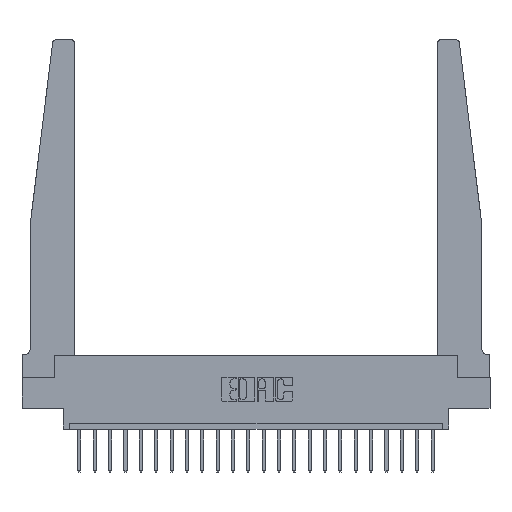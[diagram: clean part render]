
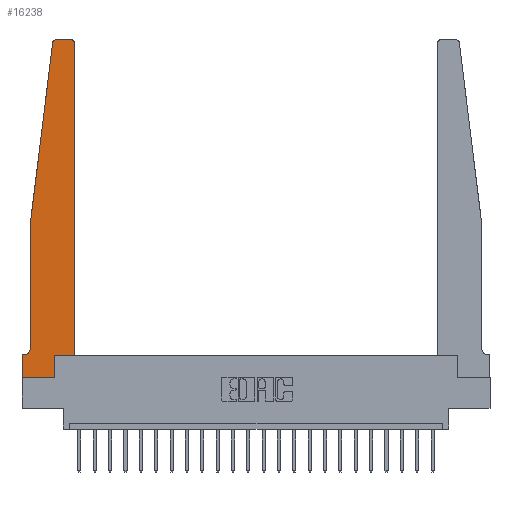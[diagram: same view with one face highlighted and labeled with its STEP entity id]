
A CAD part, top view. The second image highlights one B-rep face of the part: STEP entity #16238.
In plain terms, the highlighted planar face has unit normal (0, 0, 1).
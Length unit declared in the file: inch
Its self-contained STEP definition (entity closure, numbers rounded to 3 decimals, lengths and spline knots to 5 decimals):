
#198 = CARTESIAN_POINT ( 'NONE',  ( 0.015, 0.2375, 0.37 ) ) ;
#364 = CARTESIAN_POINT ( 'NONE',  ( 0.015, 0.1875, 0.37 ) ) ;
#538 = CARTESIAN_POINT ( 'NONE',  ( 0., 0., 0.37 ) ) ;
#600 = VECTOR ( 'NONE', #3286, 39.37008 ) ;
#659 = DIRECTION ( 'NONE',  ( -1., 0., 0. ) ) ;
#666 = CARTESIAN_POINT ( 'NONE',  ( 0.2605, 0.18, 0.37 ) ) ;
#715 = DIRECTION ( 'NONE',  ( 0., 0., 1. ) ) ;
#872 = ORIENTED_EDGE ( 'NONE', *, *, #12232, .T. ) ;
#929 = ORIENTED_EDGE ( 'NONE', *, *, #10654, .T. ) ;
#946 = CARTESIAN_POINT ( 'NONE',  ( 0.425, 0.18, 0.37 ) ) ;
#1233 = CARTESIAN_POINT ( 'NONE',  ( 0., 0., 0.37 ) ) ;
#1246 = CIRCLE ( 'NONE', #12226, 0.03 ) ;
#1289 = VECTOR ( 'NONE', #13585, 39.37008 ) ;
#1361 = CARTESIAN_POINT ( 'NONE',  ( 0.395, 2.75, 0.37 ) ) ;
#2109 = CARTESIAN_POINT ( 'NONE',  ( 0.065, 1.25, 0.37 ) ) ;
#2421 = DIRECTION ( 'NONE',  ( 1., 0., 0. ) ) ;
#2498 = DIRECTION ( 'NONE',  ( 0., 1., 0. ) ) ;
#2723 = ORIENTED_EDGE ( 'NONE', *, *, #3501, .T. ) ;
#3271 = CARTESIAN_POINT ( 'NONE',  ( 0.065, 1.25, 0.37 ) ) ;
#3286 = DIRECTION ( 'NONE',  ( 1., 0., 0. ) ) ;
#3501 = EDGE_CURVE ( 'NONE', #21080, #10775, #15341, .T. ) ;
#3715 = CARTESIAN_POINT ( 'NONE',  ( 0.395, 2.72, 0.37 ) ) ;
#3867 = DIRECTION ( 'NONE',  ( 0., 0., -1. ) ) ;
#3941 = EDGE_CURVE ( 'NONE', #10124, #15934, #20706, .T. ) ;
#4116 = CARTESIAN_POINT ( 'NONE',  ( 0.2605, 0., 0.37 ) ) ;
#4182 = CIRCLE ( 'NONE', #19936, 0.03 ) ;
#4541 = VECTOR ( 'NONE', #10244, 39.37008 ) ;
#4709 = ORIENTED_EDGE ( 'NONE', *, *, #15875, .T. ) ;
#4868 = CARTESIAN_POINT ( 'NONE',  ( 0.425, 0.18, 0.37 ) ) ;
#4977 = CARTESIAN_POINT ( 'NONE',  ( 0.425, 0.18, 0.37 ) ) ;
#5013 = DIRECTION ( 'NONE',  ( 0., -1., 0. ) ) ;
#5187 = DIRECTION ( 'NONE',  ( 1., 0., 0. ) ) ;
#5736 = CARTESIAN_POINT ( 'NONE',  ( 0.065, 0.2375, 0.37 ) ) ;
#5769 = EDGE_CURVE ( 'NONE', #15934, #6411, #4182, .T. ) ;
#5777 = CARTESIAN_POINT ( 'NONE',  ( 0.25, 2.75, 0.37 ) ) ;
#6395 = EDGE_CURVE ( 'NONE', #18772, #19838, #18056, .T. ) ;
#6411 = VERTEX_POINT ( 'NONE', #1361 ) ;
#6445 = EDGE_CURVE ( 'NONE', #16735, #21080, #10162, .T. ) ;
#6631 = ORIENTED_EDGE ( 'NONE', *, *, #19994, .T. ) ;
#6645 = VERTEX_POINT ( 'NONE', #15446 ) ;
#6826 = ORIENTED_EDGE ( 'NONE', *, *, #6395, .T. ) ;
#6922 = VECTOR ( 'NONE', #19562, 39.37008 ) ;
#7030 = EDGE_LOOP ( 'NONE', ( #4709, #20001, #929, #6631, #14098, #20085, #2723, #872, #6826, #9882, #8824, #18214 ) ) ;
#7211 = EDGE_CURVE ( 'NONE', #6645, #12249, #1246, .T. ) ;
#7307 = CARTESIAN_POINT ( 'NONE',  ( 0.065, 1.25, 0.37 ) ) ;
#8092 = CARTESIAN_POINT ( 'NONE',  ( 0., 0.1875, 0.37 ) ) ;
#8280 = EDGE_CURVE ( 'NONE', #19838, #10124, #18859, .T. ) ;
#8742 = DIRECTION ( 'NONE',  ( 0., 0., 1. ) ) ;
#8824 = ORIENTED_EDGE ( 'NONE', *, *, #3941, .T. ) ;
#9199 = EDGE_CURVE ( 'NONE', #10140, #16735, #17392, .T. ) ;
#9515 = AXIS2_PLACEMENT_3D ( 'NONE', #15859, #17453, #12198 ) ;
#9882 = ORIENTED_EDGE ( 'NONE', *, *, #8280, .T. ) ;
#9990 = VERTEX_POINT ( 'NONE', #2109 ) ;
#10124 = VERTEX_POINT ( 'NONE', #946 ) ;
#10140 = VERTEX_POINT ( 'NONE', #5736 ) ;
#10162 = LINE ( 'NONE', #18993, #10709 ) ;
#10244 = DIRECTION ( 'NONE',  ( 0., -1., 0. ) ) ;
#10272 = DIRECTION ( 'NONE',  ( -1., 0., 0. ) ) ;
#10654 = EDGE_CURVE ( 'NONE', #12249, #9990, #12238, .T. ) ;
#10709 = VECTOR ( 'NONE', #10272, 39.37008 ) ;
#10775 = VERTEX_POINT ( 'NONE', #538 ) ;
#10818 = FACE_OUTER_BOUND ( 'NONE', #7030, .T. ) ;
#11543 = AXIS2_PLACEMENT_3D ( 'NONE', #198, #3867, #659 ) ;
#11812 = VECTOR ( 'NONE', #2498, 39.37008 ) ;
#11984 = DIRECTION ( 'NONE',  ( 0., 1., 0. ) ) ;
#12198 = DIRECTION ( 'NONE',  ( 1., 0., 0. ) ) ;
#12226 = AXIS2_PLACEMENT_3D ( 'NONE', #19854, #715, #2421 ) ;
#12232 = EDGE_CURVE ( 'NONE', #10775, #18772, #18986, .T. ) ;
#12238 = LINE ( 'NONE', #7307, #13034 ) ;
#12249 = VERTEX_POINT ( 'NONE', #22535 ) ;
#12424 = PLANE ( 'NONE',  #9515 ) ;
#13034 = VECTOR ( 'NONE', #17498, 39.37008 ) ;
#13585 = DIRECTION ( 'NONE',  ( 1., 0., 0. ) ) ;
#14098 = ORIENTED_EDGE ( 'NONE', *, *, #9199, .T. ) ;
#14279 = LINE ( 'NONE', #5777, #6922 ) ;
#14568 = VECTOR ( 'NONE', #11984, 39.37008 ) ;
#15341 = LINE ( 'NONE', #17277, #18631 ) ;
#15446 = CARTESIAN_POINT ( 'NONE',  ( 0.27653, 2.75, 0.37 ) ) ;
#15513 = LINE ( 'NONE', #3271, #4541 ) ;
#15859 = CARTESIAN_POINT ( 'NONE',  ( 0., 0.1875, 0.37 ) ) ;
#15875 = EDGE_CURVE ( 'NONE', #6411, #6645, #14279, .T. ) ;
#15934 = VERTEX_POINT ( 'NONE', #16447 ) ;
#16238 = ADVANCED_FACE ( 'NONE', ( #10818 ), #12424, .T. ) ;
#16443 = CARTESIAN_POINT ( 'NONE',  ( 0.2605, 0.18, 0.37 ) ) ;
#16447 = CARTESIAN_POINT ( 'NONE',  ( 0.425, 2.72, 0.37 ) ) ;
#16735 = VERTEX_POINT ( 'NONE', #364 ) ;
#17277 = CARTESIAN_POINT ( 'NONE',  ( 0., 0., 0.37 ) ) ;
#17392 = CIRCLE ( 'NONE', #11543, 0.05 ) ;
#17453 = DIRECTION ( 'NONE',  ( 0., 0., 1. ) ) ;
#17498 = DIRECTION ( 'NONE',  ( -0.122, -0.992, 0. ) ) ;
#18056 = LINE ( 'NONE', #666, #11812 ) ;
#18214 = ORIENTED_EDGE ( 'NONE', *, *, #5769, .T. ) ;
#18631 = VECTOR ( 'NONE', #5013, 39.37008 ) ;
#18772 = VERTEX_POINT ( 'NONE', #4116 ) ;
#18859 = LINE ( 'NONE', #4868, #1289 ) ;
#18986 = LINE ( 'NONE', #1233, #600 ) ;
#18993 = CARTESIAN_POINT ( 'NONE',  ( 0.065, 0.1875, 0.37 ) ) ;
#19562 = DIRECTION ( 'NONE',  ( -1., 0., 0. ) ) ;
#19838 = VERTEX_POINT ( 'NONE', #16443 ) ;
#19854 = CARTESIAN_POINT ( 'NONE',  ( 0.27653, 2.72, 0.37 ) ) ;
#19936 = AXIS2_PLACEMENT_3D ( 'NONE', #3715, #8742, #5187 ) ;
#19994 = EDGE_CURVE ( 'NONE', #9990, #10140, #15513, .T. ) ;
#20001 = ORIENTED_EDGE ( 'NONE', *, *, #7211, .T. ) ;
#20085 = ORIENTED_EDGE ( 'NONE', *, *, #6445, .T. ) ;
#20706 = LINE ( 'NONE', #4977, #14568 ) ;
#21080 = VERTEX_POINT ( 'NONE', #8092 ) ;
#22535 = CARTESIAN_POINT ( 'NONE',  ( 0.24675, 2.72367, 0.37 ) ) ;
